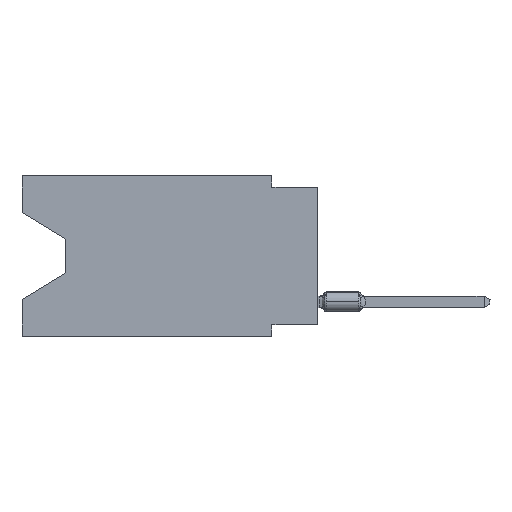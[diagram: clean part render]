
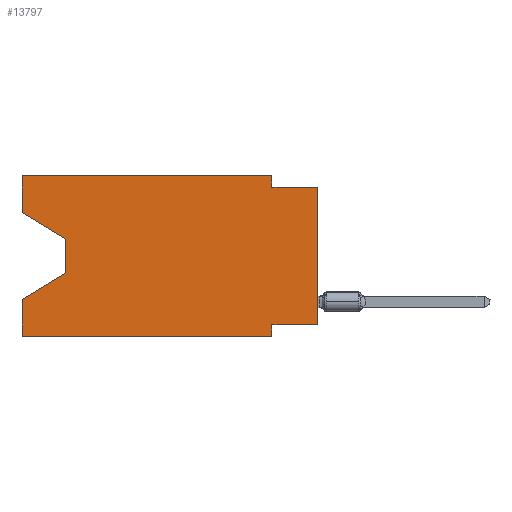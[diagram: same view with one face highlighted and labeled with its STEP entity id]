
A CAD part, left-side view. The second image highlights one B-rep face of the part: STEP entity #13797.
In plain terms, the highlighted planar face has unit normal (-1, 0, 0).
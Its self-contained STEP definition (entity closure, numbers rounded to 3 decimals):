
#623 = EDGE_CURVE ( 'NONE', #20545, #2485, #12738, .T. ) ;
#875 = CARTESIAN_POINT ( 'NONE',  ( 0., 13.97, -5.385 ) ) ;
#995 = EDGE_CURVE ( 'NONE', #36294, #21816, #32108, .T. ) ;
#1282 = PLANE ( 'NONE',  #2525 ) ;
#1333 = CARTESIAN_POINT ( 'NONE',  ( 0., 2.54, 0. ) ) ;
#2485 = VERTEX_POINT ( 'NONE', #30007 ) ;
#2525 = AXIS2_PLACEMENT_3D ( 'NONE', #10756, #10961, #5023 ) ;
#2934 = LINE ( 'NONE', #38530, #32308 ) ;
#3061 = VERTEX_POINT ( 'NONE', #26372 ) ;
#3486 = EDGE_CURVE ( 'NONE', #3061, #2485, #16353, .T. ) ;
#4071 = VECTOR ( 'NONE', #18173, 1000. ) ;
#4618 = LINE ( 'NONE', #16672, #18412 ) ;
#4748 = ORIENTED_EDGE ( 'NONE', *, *, #995, .F. ) ;
#4834 = VECTOR ( 'NONE', #38489, 1000. ) ;
#4975 = DIRECTION ( 'NONE',  ( 0., -1., 0. ) ) ;
#5023 = DIRECTION ( 'NONE',  ( 0., 0., -1. ) ) ;
#5041 = DIRECTION ( 'NONE',  ( 0., 0., 1. ) ) ;
#5342 = DIRECTION ( 'NONE',  ( 0., -0.855, -0.519 ) ) ;
#6193 = ORIENTED_EDGE ( 'NONE', *, *, #39091, .T. ) ;
#6247 = EDGE_LOOP ( 'NONE', ( #26539, #6193, #20296, #20388, #12623, #8983, #31505, #32332, #32260, #38476, #35836, #4748 ) ) ;
#6485 = DIRECTION ( 'NONE',  ( 0., -1., 0. ) ) ;
#6585 = VECTOR ( 'NONE', #5041, 1000. ) ;
#7315 = DIRECTION ( 'NONE',  ( 0., 0., 1. ) ) ;
#7647 = VERTEX_POINT ( 'NONE', #26881 ) ;
#8920 = VERTEX_POINT ( 'NONE', #28086 ) ;
#8983 = ORIENTED_EDGE ( 'NONE', *, *, #19025, .F. ) ;
#9575 = DIRECTION ( 'NONE',  ( 0., 0.855, -0.519 ) ) ;
#10400 = CARTESIAN_POINT ( 'NONE',  ( 0., 16.383, 0. ) ) ;
#10756 = CARTESIAN_POINT ( 'NONE',  ( 0., 16.383, 0. ) ) ;
#10961 = DIRECTION ( 'NONE',  ( 1., 0., 0. ) ) ;
#11330 = CARTESIAN_POINT ( 'NONE',  ( 0., 16.383, 0. ) ) ;
#11949 = VERTEX_POINT ( 'NONE', #13300 ) ;
#12623 = ORIENTED_EDGE ( 'NONE', *, *, #32250, .T. ) ;
#12738 = LINE ( 'NONE', #875, #31504 ) ;
#13261 = VERTEX_POINT ( 'NONE', #36125 ) ;
#13300 = CARTESIAN_POINT ( 'NONE',  ( 0., 0., -8.255 ) ) ;
#13797 = ADVANCED_FACE ( 'NONE', ( #28937 ), #1282, .F. ) ;
#14234 = LINE ( 'NONE', #20143, #31021 ) ;
#14378 = LINE ( 'NONE', #37888, #4834 ) ;
#14828 = EDGE_CURVE ( 'NONE', #11949, #18392, #20983, .T. ) ;
#15061 = EDGE_CURVE ( 'NONE', #36294, #8920, #14234, .T. ) ;
#15529 = LINE ( 'NONE', #15717, #34480 ) ;
#15717 = CARTESIAN_POINT ( 'NONE',  ( 0., 2.54, 0. ) ) ;
#15745 = CARTESIAN_POINT ( 'NONE',  ( 0., 2.54, -8.255 ) ) ;
#16353 = LINE ( 'NONE', #30969, #30082 ) ;
#16468 = VECTOR ( 'NONE', #18020, 1000. ) ;
#16672 = CARTESIAN_POINT ( 'NONE',  ( 0., 2.54, -8.89 ) ) ;
#16878 = EDGE_CURVE ( 'NONE', #11949, #22644, #32552, .T. ) ;
#18020 = DIRECTION ( 'NONE',  ( 0., 1., 0. ) ) ;
#18173 = DIRECTION ( 'NONE',  ( 0., -1., 0. ) ) ;
#18392 = VERTEX_POINT ( 'NONE', #15745 ) ;
#18412 = VECTOR ( 'NONE', #28724, 1000. ) ;
#19025 = EDGE_CURVE ( 'NONE', #18392, #7647, #4618, .T. ) ;
#20143 = CARTESIAN_POINT ( 'NONE',  ( 0., 16.383, -2.038 ) ) ;
#20296 = ORIENTED_EDGE ( 'NONE', *, *, #623, .T. ) ;
#20388 = ORIENTED_EDGE ( 'NONE', *, *, #3486, .F. ) ;
#20545 = VERTEX_POINT ( 'NONE', #30717 ) ;
#20840 = EDGE_CURVE ( 'NONE', #13261, #22644, #27866, .T. ) ;
#20983 = LINE ( 'NONE', #36197, #16468 ) ;
#21816 = VERTEX_POINT ( 'NONE', #11330 ) ;
#22644 = VERTEX_POINT ( 'NONE', #32533 ) ;
#23660 = CARTESIAN_POINT ( 'NONE',  ( 0., 0., 0. ) ) ;
#25565 = CARTESIAN_POINT ( 'NONE',  ( 0., 16.383, 0. ) ) ;
#26372 = CARTESIAN_POINT ( 'NONE',  ( 0., 16.383, -8.89 ) ) ;
#26374 = VECTOR ( 'NONE', #4975, 1000. ) ;
#26539 = ORIENTED_EDGE ( 'NONE', *, *, #15061, .T. ) ;
#26881 = CARTESIAN_POINT ( 'NONE',  ( 0., 2.54, -8.89 ) ) ;
#27866 = LINE ( 'NONE', #36155, #4071 ) ;
#28086 = CARTESIAN_POINT ( 'NONE',  ( 0., 13.97, -3.505 ) ) ;
#28226 = DIRECTION ( 'NONE',  ( 0., 0., 1. ) ) ;
#28233 = EDGE_CURVE ( 'NONE', #21816, #32517, #37402, .T. ) ;
#28724 = DIRECTION ( 'NONE',  ( 0., 0., -1. ) ) ;
#28937 = FACE_OUTER_BOUND ( 'NONE', #6247, .T. ) ;
#29547 = EDGE_CURVE ( 'NONE', #32517, #13261, #15529, .T. ) ;
#30007 = CARTESIAN_POINT ( 'NONE',  ( 0., 16.383, -6.852 ) ) ;
#30082 = VECTOR ( 'NONE', #28226, 1000. ) ;
#30544 = DIRECTION ( 'NONE',  ( 0., 0., -1. ) ) ;
#30717 = CARTESIAN_POINT ( 'NONE',  ( 0., 13.97, -5.385 ) ) ;
#30969 = CARTESIAN_POINT ( 'NONE',  ( 0., 16.383, 0. ) ) ;
#31021 = VECTOR ( 'NONE', #5342, 1000. ) ;
#31504 = VECTOR ( 'NONE', #9575, 1000. ) ;
#31505 = ORIENTED_EDGE ( 'NONE', *, *, #14828, .F. ) ;
#32108 = LINE ( 'NONE', #10400, #6585 ) ;
#32250 = EDGE_CURVE ( 'NONE', #3061, #7647, #2934, .T. ) ;
#32260 = ORIENTED_EDGE ( 'NONE', *, *, #20840, .F. ) ;
#32308 = VECTOR ( 'NONE', #6485, 1000. ) ;
#32332 = ORIENTED_EDGE ( 'NONE', *, *, #16878, .T. ) ;
#32517 = VERTEX_POINT ( 'NONE', #1333 ) ;
#32533 = CARTESIAN_POINT ( 'NONE',  ( 0., 0., -0.635 ) ) ;
#32552 = LINE ( 'NONE', #23660, #38494 ) ;
#34480 = VECTOR ( 'NONE', #30544, 1000. ) ;
#35836 = ORIENTED_EDGE ( 'NONE', *, *, #28233, .F. ) ;
#36125 = CARTESIAN_POINT ( 'NONE',  ( 0., 2.54, -0.635 ) ) ;
#36155 = CARTESIAN_POINT ( 'NONE',  ( 0., 0., -0.635 ) ) ;
#36197 = CARTESIAN_POINT ( 'NONE',  ( 0., 0., -8.255 ) ) ;
#36294 = VERTEX_POINT ( 'NONE', #38897 ) ;
#37402 = LINE ( 'NONE', #25565, #26374 ) ;
#37888 = CARTESIAN_POINT ( 'NONE',  ( 0., 13.97, -3.505 ) ) ;
#38476 = ORIENTED_EDGE ( 'NONE', *, *, #29547, .F. ) ;
#38489 = DIRECTION ( 'NONE',  ( 0., 0., -1. ) ) ;
#38494 = VECTOR ( 'NONE', #7315, 1000. ) ;
#38530 = CARTESIAN_POINT ( 'NONE',  ( 0., 16.383, -8.89 ) ) ;
#38897 = CARTESIAN_POINT ( 'NONE',  ( 0., 16.383, -2.038 ) ) ;
#39091 = EDGE_CURVE ( 'NONE', #8920, #20545, #14378, .T. ) ;
